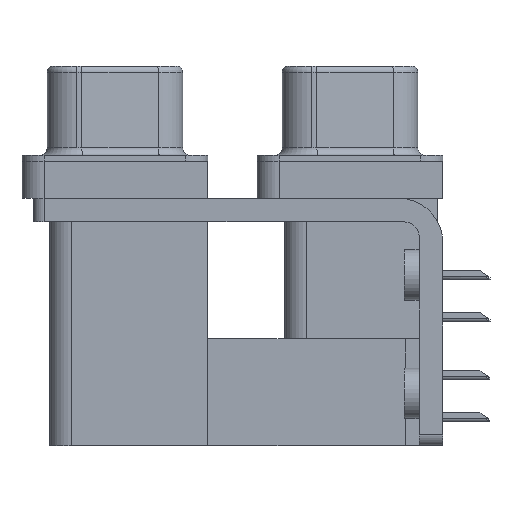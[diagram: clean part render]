
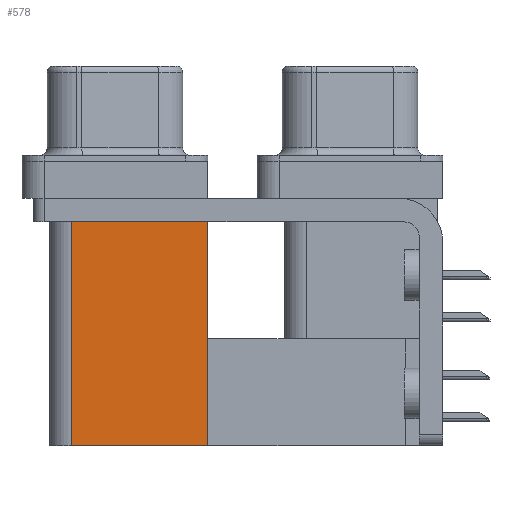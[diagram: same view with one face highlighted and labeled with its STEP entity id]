
A CAD part, left-side view. The second image highlights one B-rep face of the part: STEP entity #578.
In plain terms, the highlighted planar face has unit normal (-1, 0, 0).
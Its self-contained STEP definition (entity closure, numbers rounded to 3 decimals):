
#382 = VERTEX_POINT ( 'NONE', #6742 ) ;
#578 = ADVANCED_FACE ( 'NONE', ( #1918 ), #20220, .F. ) ;
#1087 = CARTESIAN_POINT ( 'NONE',  ( 3.765, 9.6, -19.2 ) ) ;
#1918 = FACE_OUTER_BOUND ( 'NONE', #9323, .T. ) ;
#4979 = CARTESIAN_POINT ( 'NONE',  ( 3.765, 18.8, -19.2 ) ) ;
#6742 = CARTESIAN_POINT ( 'NONE',  ( 3.765, 9.6, -19.2 ) ) ;
#7560 = VECTOR ( 'NONE', #27721, 1000. ) ;
#7736 = VERTEX_POINT ( 'NONE', #18286 ) ;
#7940 = LINE ( 'NONE', #8276, #30305 ) ;
#8276 = CARTESIAN_POINT ( 'NONE',  ( 3.765, 9.6, -19.2 ) ) ;
#9323 = EDGE_LOOP ( 'NONE', ( #30172, #16031, #10555, #27117 ) ) ;
#10555 = ORIENTED_EDGE ( 'NONE', *, *, #28834, .F. ) ;
#12154 = LINE ( 'NONE', #4979, #7560 ) ;
#12183 = DIRECTION ( 'NONE',  ( 1., 0., 0. ) ) ;
#12283 = CARTESIAN_POINT ( 'NONE',  ( 3.765, 18.8, -2.5 ) ) ;
#14754 = CARTESIAN_POINT ( 'NONE',  ( 3.765, 9.6, -19.2 ) ) ;
#16031 = ORIENTED_EDGE ( 'NONE', *, *, #25701, .F. ) ;
#16347 = DIRECTION ( 'NONE',  ( 0., 1., 0. ) ) ;
#17252 = VECTOR ( 'NONE', #16347, 1000. ) ;
#17858 = VERTEX_POINT ( 'NONE', #21506 ) ;
#18257 = VECTOR ( 'NONE', #19224, 1000. ) ;
#18286 = CARTESIAN_POINT ( 'NONE',  ( 3.765, 18.8, -19.2 ) ) ;
#19224 = DIRECTION ( 'NONE',  ( 0., 0., 1. ) ) ;
#19404 = LINE ( 'NONE', #26935, #17252 ) ;
#20220 = PLANE ( 'NONE',  #26370 ) ;
#21265 = EDGE_CURVE ( 'NONE', #382, #17858, #24496, .T. ) ;
#21506 = CARTESIAN_POINT ( 'NONE',  ( 3.765, 9.6, -2.5 ) ) ;
#22600 = DIRECTION ( 'NONE',  ( 0., 0., -1. ) ) ;
#24496 = LINE ( 'NONE', #1087, #18257 ) ;
#25701 = EDGE_CURVE ( 'NONE', #7736, #32936, #12154, .T. ) ;
#26370 = AXIS2_PLACEMENT_3D ( 'NONE', #14754, #12183, #22600 ) ;
#26935 = CARTESIAN_POINT ( 'NONE',  ( 3.765, 9.6, -2.5 ) ) ;
#27117 = ORIENTED_EDGE ( 'NONE', *, *, #21265, .T. ) ;
#27721 = DIRECTION ( 'NONE',  ( 0., 0., 1. ) ) ;
#28834 = EDGE_CURVE ( 'NONE', #382, #7736, #7940, .T. ) ;
#30172 = ORIENTED_EDGE ( 'NONE', *, *, #31795, .T. ) ;
#30305 = VECTOR ( 'NONE', #31990, 1000. ) ;
#31795 = EDGE_CURVE ( 'NONE', #17858, #32936, #19404, .T. ) ;
#31990 = DIRECTION ( 'NONE',  ( 0., 1., 0. ) ) ;
#32936 = VERTEX_POINT ( 'NONE', #12283 ) ;
